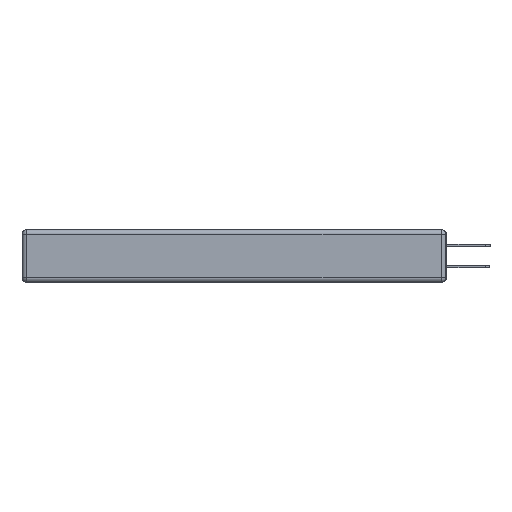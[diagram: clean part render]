
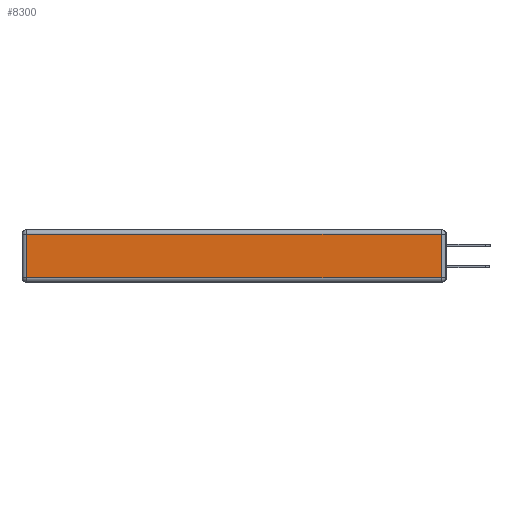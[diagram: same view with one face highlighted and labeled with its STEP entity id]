
A CAD part, left-side view. The second image highlights one B-rep face of the part: STEP entity #8300.
In plain terms, the highlighted planar face has unit normal (-1, 0, 0).
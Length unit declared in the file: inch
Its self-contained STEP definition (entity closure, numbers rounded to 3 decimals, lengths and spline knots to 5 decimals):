
#139 = VERTEX_POINT ( 'NONE', #21722 ) ;
#550 = LINE ( 'NONE', #18842, #8095 ) ;
#910 = ORIENTED_EDGE ( 'NONE', *, *, #22156, .T. ) ;
#2606 = CARTESIAN_POINT ( 'NONE',  ( 0., 0., -0.343 ) ) ;
#3035 = LINE ( 'NONE', #3718, #14565 ) ;
#3678 = DIRECTION ( 'NONE',  ( 0., 0., -1. ) ) ;
#3718 = CARTESIAN_POINT ( 'NONE',  ( 0., 0., -0.313 ) ) ;
#4240 = CARTESIAN_POINT ( 'NONE',  ( 0., 0.03, -0.343 ) ) ;
#4543 = EDGE_CURVE ( 'NONE', #19859, #11522, #11856, .T. ) ;
#7030 = AXIS2_PLACEMENT_3D ( 'NONE', #2606, #7720, #7860 ) ;
#7720 = DIRECTION ( 'NONE',  ( -1., 0., 0. ) ) ;
#7860 = DIRECTION ( 'NONE',  ( 0., 0., 1. ) ) ;
#8095 = VECTOR ( 'NONE', #16793, 39.37008 ) ;
#8300 = ADVANCED_FACE ( 'NONE', ( #8970 ), #19795, .T. ) ;
#8970 = FACE_OUTER_BOUND ( 'NONE', #15213, .T. ) ;
#11522 = VERTEX_POINT ( 'NONE', #20728 ) ;
#11856 = LINE ( 'NONE', #15433, #16405 ) ;
#12103 = CARTESIAN_POINT ( 'NONE',  ( 0., 2.72, -0.03 ) ) ;
#12573 = ORIENTED_EDGE ( 'NONE', *, *, #15741, .T. ) ;
#12671 = VECTOR ( 'NONE', #19622, 39.37008 ) ;
#12838 = DIRECTION ( 'NONE',  ( 0., -1., 0. ) ) ;
#12941 = LINE ( 'NONE', #4240, #12671 ) ;
#13544 = ORIENTED_EDGE ( 'NONE', *, *, #4543, .T. ) ;
#13668 = EDGE_CURVE ( 'NONE', #11522, #139, #3035, .T. ) ;
#14565 = VECTOR ( 'NONE', #12838, 39.37008 ) ;
#14672 = VERTEX_POINT ( 'NONE', #21961 ) ;
#15213 = EDGE_LOOP ( 'NONE', ( #16315, #910, #12573, #13544 ) ) ;
#15433 = CARTESIAN_POINT ( 'NONE',  ( 0., 2.72, -0.343 ) ) ;
#15741 = EDGE_CURVE ( 'NONE', #14672, #19859, #550, .T. ) ;
#16315 = ORIENTED_EDGE ( 'NONE', *, *, #13668, .T. ) ;
#16405 = VECTOR ( 'NONE', #3678, 39.37008 ) ;
#16793 = DIRECTION ( 'NONE',  ( 0., 1., 0. ) ) ;
#18842 = CARTESIAN_POINT ( 'NONE',  ( 0., 2.75, -0.03 ) ) ;
#19622 = DIRECTION ( 'NONE',  ( 0., 0., 1. ) ) ;
#19795 = PLANE ( 'NONE',  #7030 ) ;
#19859 = VERTEX_POINT ( 'NONE', #12103 ) ;
#20728 = CARTESIAN_POINT ( 'NONE',  ( 0., 2.72, -0.313 ) ) ;
#21722 = CARTESIAN_POINT ( 'NONE',  ( 0., 0.03, -0.313 ) ) ;
#21961 = CARTESIAN_POINT ( 'NONE',  ( 0., 0.03, -0.03 ) ) ;
#22156 = EDGE_CURVE ( 'NONE', #139, #14672, #12941, .T. ) ;
